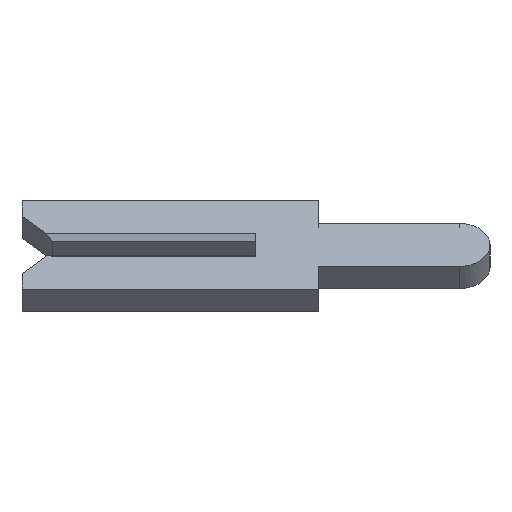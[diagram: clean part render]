
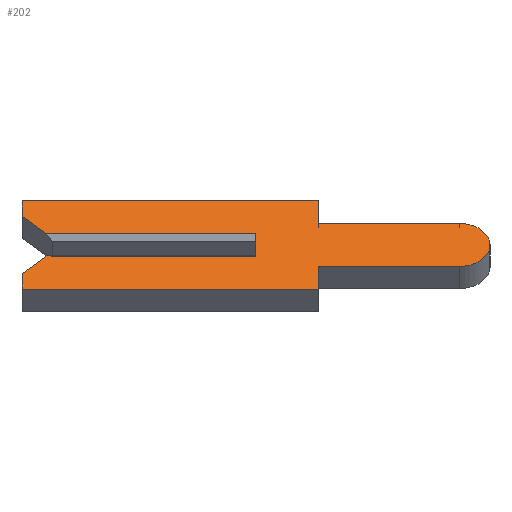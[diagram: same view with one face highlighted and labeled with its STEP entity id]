
A CAD part, left-side view. The second image highlights one B-rep face of the part: STEP entity #202.
In plain terms, the highlighted face is planar.
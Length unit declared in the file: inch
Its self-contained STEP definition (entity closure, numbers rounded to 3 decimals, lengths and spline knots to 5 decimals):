
#1 = VECTOR ( 'NONE', #581, 39.37008 ) ;
#2 = CARTESIAN_POINT ( 'NONE',  ( -0.01, 0.15, 0.01 ) ) ;
#15 = CARTESIAN_POINT ( 'NONE',  ( -0.01, -0.04, 0.04 ) ) ;
#16 = VERTEX_POINT ( 'NONE', #851 ) ;
#17 = VECTOR ( 'NONE', #248, 39.37008 ) ;
#41 = VERTEX_POINT ( 'NONE', #871 ) ;
#51 = ORIENTED_EDGE ( 'NONE', *, *, #872, .F. ) ;
#69 = DIRECTION ( 'NONE',  ( 0., 0., 1. ) ) ;
#148 = ORIENTED_EDGE ( 'NONE', *, *, #547, .F. ) ;
#149 = CARTESIAN_POINT ( 'NONE',  ( -0.01, -0.1305, 0. ) ) ;
#156 = CARTESIAN_POINT ( 'NONE',  ( -0.01, 0.15, -0.04 ) ) ;
#163 = EDGE_CURVE ( 'NONE', #505, #596, #801, .T. ) ;
#172 = LINE ( 'NONE', #1199, #1004 ) ;
#185 = DIRECTION ( 'NONE',  ( 1., 0., 0. ) ) ;
#191 = VECTOR ( 'NONE', #1091, 39.37008 ) ;
#192 = ORIENTED_EDGE ( 'NONE', *, *, #533, .F. ) ;
#194 = EDGE_CURVE ( 'NONE', #41, #505, #665, .T. ) ;
#202 = ADVANCED_FACE ( 'NONE', ( #1223 ), #770, .F. ) ;
#206 = CARTESIAN_POINT ( 'NONE',  ( -0.01, 0.15, -0.026 ) ) ;
#223 = CARTESIAN_POINT ( 'NONE',  ( -0.01, -0.04, -0.04 ) ) ;
#242 = ORIENTED_EDGE ( 'NONE', *, *, #414, .F. ) ;
#248 = DIRECTION ( 'NONE',  ( 0., 1., 0. ) ) ;
#255 = VERTEX_POINT ( 'NONE', #768 ) ;
#263 = VERTEX_POINT ( 'NONE', #373 ) ;
#268 = CARTESIAN_POINT ( 'NONE',  ( -0.01, -0.1305, 0. ) ) ;
#272 = DIRECTION ( 'NONE',  ( 1., 0., 0. ) ) ;
#280 = LINE ( 'NONE', #156, #298 ) ;
#281 = DIRECTION ( 'NONE',  ( 0., -1., 0. ) ) ;
#287 = DIRECTION ( 'NONE',  ( 0., 0., -1. ) ) ;
#296 = CARTESIAN_POINT ( 'NONE',  ( -0.01, -0.1305, -0.01 ) ) ;
#298 = VECTOR ( 'NONE', #1158, 39.37008 ) ;
#373 = CARTESIAN_POINT ( 'NONE',  ( -0.01, 0.15, 0.04 ) ) ;
#391 = LINE ( 'NONE', #15, #1157 ) ;
#394 = CARTESIAN_POINT ( 'NONE',  ( -0.01, 0.134, -0.01 ) ) ;
#406 = LINE ( 'NONE', #439, #17 ) ;
#414 = EDGE_CURVE ( 'NONE', #263, #847, #593, .T. ) ;
#425 = ORIENTED_EDGE ( 'NONE', *, *, #946, .F. ) ;
#438 = EDGE_CURVE ( 'NONE', #1066, #263, #1063, .T. ) ;
#439 = CARTESIAN_POINT ( 'NONE',  ( -0.01, -0.04, -0.0195 ) ) ;
#450 = VERTEX_POINT ( 'NONE', #1094 ) ;
#469 = LINE ( 'NONE', #893, #191 ) ;
#486 = CARTESIAN_POINT ( 'NONE',  ( -0.01, 0.15, 0.026 ) ) ;
#487 = VERTEX_POINT ( 'NONE', #773 ) ;
#495 = CARTESIAN_POINT ( 'NONE',  ( -0.01, 0., 0.01 ) ) ;
#499 = CARTESIAN_POINT ( 'NONE',  ( -0.01, -0.1305, -0.0195 ) ) ;
#501 = VERTEX_POINT ( 'NONE', #791 ) ;
#505 = VERTEX_POINT ( 'NONE', #206 ) ;
#531 = ORIENTED_EDGE ( 'NONE', *, *, #800, .F. ) ;
#533 = EDGE_CURVE ( 'NONE', #501, #908, #172, .T. ) ;
#539 = AXIS2_PLACEMENT_3D ( 'NONE', #268, #185, #287 ) ;
#547 = EDGE_CURVE ( 'NONE', #255, #1066, #469, .T. ) ;
#548 = VECTOR ( 'NONE', #1188, 39.37008 ) ;
#551 = VERTEX_POINT ( 'NONE', #495 ) ;
#552 = CARTESIAN_POINT ( 'NONE',  ( -0.01, 0.15, 0.026 ) ) ;
#573 = ORIENTED_EDGE ( 'NONE', *, *, #922, .F. ) ;
#581 = DIRECTION ( 'NONE',  ( 0., -0.707, 0.707 ) ) ;
#593 = LINE ( 'NONE', #862, #913 ) ;
#596 = VERTEX_POINT ( 'NONE', #394 ) ;
#623 = DIRECTION ( 'NONE',  ( 0., 0., -1. ) ) ;
#629 = CARTESIAN_POINT ( 'NONE',  ( -0.01, 0., 0.0065 ) ) ;
#630 = LINE ( 'NONE', #629, #1026 ) ;
#632 = EDGE_CURVE ( 'NONE', #596, #487, #1036, .T. ) ;
#635 = DIRECTION ( 'NONE',  ( 0., 0., 1. ) ) ;
#654 = EDGE_CURVE ( 'NONE', #255, #551, #1017, .T. ) ;
#663 = VERTEX_POINT ( 'NONE', #499 ) ;
#665 = LINE ( 'NONE', #857, #743 ) ;
#711 = CARTESIAN_POINT ( 'NONE',  ( -0.01, -0.04, 0.04 ) ) ;
#743 = VECTOR ( 'NONE', #69, 39.37008 ) ;
#757 = VECTOR ( 'NONE', #883, 39.37008 ) ;
#768 = CARTESIAN_POINT ( 'NONE',  ( -0.01, 0.134, 0.01 ) ) ;
#770 = PLANE ( 'NONE',  #539 ) ;
#773 = CARTESIAN_POINT ( 'NONE',  ( -0.01, 0., -0.01 ) ) ;
#783 = ORIENTED_EDGE ( 'NONE', *, *, #632, .F. ) ;
#791 = CARTESIAN_POINT ( 'NONE',  ( -0.01, -0.04, -0.0195 ) ) ;
#800 = EDGE_CURVE ( 'NONE', #16, #450, #1236, .T. ) ;
#801 = LINE ( 'NONE', #1177, #1 ) ;
#806 = CARTESIAN_POINT ( 'NONE',  ( -0.01, -0.04, 0.0195 ) ) ;
#839 = ORIENTED_EDGE ( 'NONE', *, *, #194, .F. ) ;
#847 = VERTEX_POINT ( 'NONE', #711 ) ;
#851 = CARTESIAN_POINT ( 'NONE',  ( -0.01, -0.04, 0.0195 ) ) ;
#857 = CARTESIAN_POINT ( 'NONE',  ( -0.01, 0.15, -0.026 ) ) ;
#862 = CARTESIAN_POINT ( 'NONE',  ( -0.01, 0.15, 0.04 ) ) ;
#871 = CARTESIAN_POINT ( 'NONE',  ( -0.01, 0.15, -0.04 ) ) ;
#872 = EDGE_CURVE ( 'NONE', #847, #16, #391, .T. ) ;
#883 = DIRECTION ( 'NONE',  ( 0., -1., 0. ) ) ;
#891 = CIRCLE ( 'NONE', #1080, 0.0195 ) ;
#893 = CARTESIAN_POINT ( 'NONE',  ( -0.01, 0.1305, 0.0065 ) ) ;
#908 = VERTEX_POINT ( 'NONE', #223 ) ;
#913 = VECTOR ( 'NONE', #281, 39.37008 ) ;
#922 = EDGE_CURVE ( 'NONE', #487, #551, #630, .T. ) ;
#928 = ORIENTED_EDGE ( 'NONE', *, *, #163, .F. ) ;
#945 = EDGE_LOOP ( 'NONE', ( #1113, #573, #783, #928, #839, #995, #192, #425, #960, #531, #51, #242, #965, #148 ) ) ;
#946 = EDGE_CURVE ( 'NONE', #663, #501, #406, .T. ) ;
#950 = DIRECTION ( 'NONE',  ( 0., 0., -1. ) ) ;
#960 = ORIENTED_EDGE ( 'NONE', *, *, #1198, .F. ) ;
#965 = ORIENTED_EDGE ( 'NONE', *, *, #438, .F. ) ;
#990 = DIRECTION ( 'NONE',  ( 0., -1., 0. ) ) ;
#995 = ORIENTED_EDGE ( 'NONE', *, *, #1258, .F. ) ;
#1004 = VECTOR ( 'NONE', #1096, 39.37008 ) ;
#1013 = DIRECTION ( 'NONE',  ( 0., -1., 0. ) ) ;
#1017 = LINE ( 'NONE', #2, #1050 ) ;
#1026 = VECTOR ( 'NONE', #635, 39.37008 ) ;
#1036 = LINE ( 'NONE', #296, #757 ) ;
#1050 = VECTOR ( 'NONE', #990, 39.37008 ) ;
#1063 = LINE ( 'NONE', #486, #548 ) ;
#1066 = VERTEX_POINT ( 'NONE', #552 ) ;
#1080 = AXIS2_PLACEMENT_3D ( 'NONE', #149, #272, #950 ) ;
#1091 = DIRECTION ( 'NONE',  ( 0., 0.707, 0.707 ) ) ;
#1094 = CARTESIAN_POINT ( 'NONE',  ( -0.01, -0.1305, 0.0195 ) ) ;
#1096 = DIRECTION ( 'NONE',  ( 0., 0., -1. ) ) ;
#1113 = ORIENTED_EDGE ( 'NONE', *, *, #654, .T. ) ;
#1144 = VECTOR ( 'NONE', #1013, 39.37008 ) ;
#1157 = VECTOR ( 'NONE', #623, 39.37008 ) ;
#1158 = DIRECTION ( 'NONE',  ( 0., 1., 0. ) ) ;
#1177 = CARTESIAN_POINT ( 'NONE',  ( -0.01, 0.1305, -0.0065 ) ) ;
#1188 = DIRECTION ( 'NONE',  ( 0., 0., 1. ) ) ;
#1198 = EDGE_CURVE ( 'NONE', #450, #663, #891, .T. ) ;
#1199 = CARTESIAN_POINT ( 'NONE',  ( -0.01, -0.04, -0.04 ) ) ;
#1223 = FACE_OUTER_BOUND ( 'NONE', #945, .T. ) ;
#1236 = LINE ( 'NONE', #806, #1144 ) ;
#1258 = EDGE_CURVE ( 'NONE', #908, #41, #280, .T. ) ;
